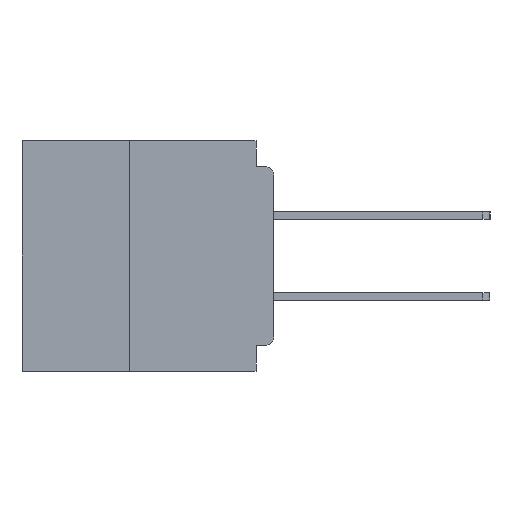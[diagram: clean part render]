
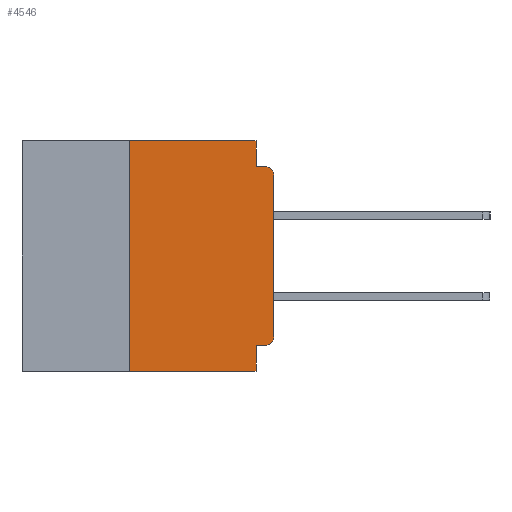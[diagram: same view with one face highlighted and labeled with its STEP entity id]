
A CAD part, left-side view. The second image highlights one B-rep face of the part: STEP entity #4546.
In plain terms, the highlighted planar face has unit normal (-1, 0, 0).
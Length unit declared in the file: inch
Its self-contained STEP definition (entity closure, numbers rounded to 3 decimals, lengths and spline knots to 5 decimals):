
#869 = EDGE_CURVE ( 'NONE', #6535, #37464, #2580, .T. ) ;
#2446 = CARTESIAN_POINT ( 'NONE',  ( 0., 0.015, -0.34 ) ) ;
#2580 = LINE ( 'NONE', #14426, #40283 ) ;
#2788 = CARTESIAN_POINT ( 'NONE',  ( 0., 0.031, -0.4 ) ) ;
#2924 = CARTESIAN_POINT ( 'NONE',  ( 0., 0., -0.045 ) ) ;
#3653 = EDGE_CURVE ( 'NONE', #5623, #40461, #44685, .T. ) ;
#4222 = DIRECTION ( 'NONE',  ( 0., 0., -1. ) ) ;
#4546 = ADVANCED_FACE ( 'NONE', ( #43431 ), #31111, .F. ) ;
#4682 = ORIENTED_EDGE ( 'NONE', *, *, #29597, .F. ) ;
#5073 = DIRECTION ( 'NONE',  ( 0., 0., 1. ) ) ;
#5623 = VERTEX_POINT ( 'NONE', #37972 ) ;
#5752 = LINE ( 'NONE', #2788, #24619 ) ;
#5848 = EDGE_CURVE ( 'NONE', #23133, #26638, #44466, .T. ) ;
#6273 = DIRECTION ( 'NONE',  ( 0., 0., -1. ) ) ;
#6535 = VERTEX_POINT ( 'NONE', #35737 ) ;
#7078 = ORIENTED_EDGE ( 'NONE', *, *, #17910, .T. ) ;
#7271 = CARTESIAN_POINT ( 'NONE',  ( 0., 0.015, -0.06 ) ) ;
#8165 = CARTESIAN_POINT ( 'NONE',  ( 0., 0.015, -0.355 ) ) ;
#8594 = DIRECTION ( 'NONE',  ( 1., 0., 0. ) ) ;
#9610 = DIRECTION ( 'NONE',  ( 0., 1., 0. ) ) ;
#9863 = ORIENTED_EDGE ( 'NONE', *, *, #44425, .F. ) ;
#10443 = LINE ( 'NONE', #32131, #40440 ) ;
#11064 = DIRECTION ( 'NONE',  ( 0., 0., -1. ) ) ;
#12725 = CARTESIAN_POINT ( 'NONE',  ( 0., 0.031, -0.045 ) ) ;
#12985 = VECTOR ( 'NONE', #4222, 39.37008 ) ;
#14413 = CARTESIAN_POINT ( 'NONE',  ( 0., 0.031, 0. ) ) ;
#14426 = CARTESIAN_POINT ( 'NONE',  ( 0., 0.437, -0.4 ) ) ;
#14863 = CIRCLE ( 'NONE', #47612, 0.015 ) ;
#15536 = EDGE_CURVE ( 'NONE', #40461, #44170, #42951, .T. ) ;
#15879 = VERTEX_POINT ( 'NONE', #25126 ) ;
#16099 = LINE ( 'NONE', #2924, #27312 ) ;
#17910 = EDGE_CURVE ( 'NONE', #26638, #42758, #18728, .T. ) ;
#18728 = CIRCLE ( 'NONE', #38274, 0.015 ) ;
#20523 = CARTESIAN_POINT ( 'NONE',  ( 0., 0., 0. ) ) ;
#21500 = CARTESIAN_POINT ( 'NONE',  ( 0., 0.437, 0. ) ) ;
#21781 = DIRECTION ( 'NONE',  ( 0., 0., -1. ) ) ;
#22965 = VECTOR ( 'NONE', #5073, 39.37008 ) ;
#23133 = VERTEX_POINT ( 'NONE', #34748 ) ;
#23736 = EDGE_LOOP ( 'NONE', ( #25271, #7078, #24298, #45502, #30914, #46798, #47444, #9863, #4682, #31792 ) ) ;
#24298 = ORIENTED_EDGE ( 'NONE', *, *, #31698, .F. ) ;
#24448 = VERTEX_POINT ( 'NONE', #8165 ) ;
#24619 = VECTOR ( 'NONE', #21781, 39.37008 ) ;
#24737 = CARTESIAN_POINT ( 'NONE',  ( 0., 0., -0.06 ) ) ;
#24789 = CARTESIAN_POINT ( 'NONE',  ( 0., 0.015, -0.045 ) ) ;
#25126 = CARTESIAN_POINT ( 'NONE',  ( 0., 0.031, -0.355 ) ) ;
#25271 = ORIENTED_EDGE ( 'NONE', *, *, #5848, .T. ) ;
#25281 = DIRECTION ( 'NONE',  ( 0., -1., 0. ) ) ;
#25521 = DIRECTION ( 'NONE',  ( 0., -1., 0. ) ) ;
#25658 = CARTESIAN_POINT ( 'NONE',  ( 0., 0.031, -0.4 ) ) ;
#25721 = VECTOR ( 'NONE', #46725, 39.37008 ) ;
#26638 = VERTEX_POINT ( 'NONE', #24737 ) ;
#27312 = VECTOR ( 'NONE', #25521, 39.37008 ) ;
#28806 = DIRECTION ( 'NONE',  ( -1., 0., 0. ) ) ;
#28875 = EDGE_CURVE ( 'NONE', #6535, #5623, #41717, .T. ) ;
#29597 = EDGE_CURVE ( 'NONE', #24448, #15879, #10443, .T. ) ;
#30914 = ORIENTED_EDGE ( 'NONE', *, *, #3653, .F. ) ;
#31111 = PLANE ( 'NONE',  #34516 ) ;
#31234 = DIRECTION ( 'NONE',  ( 0., -1., 0. ) ) ;
#31698 = EDGE_CURVE ( 'NONE', #44170, #42758, #16099, .T. ) ;
#31792 = ORIENTED_EDGE ( 'NONE', *, *, #46714, .T. ) ;
#32131 = CARTESIAN_POINT ( 'NONE',  ( 0., 0., -0.355 ) ) ;
#33562 = DIRECTION ( 'NONE',  ( -1., 0., 0. ) ) ;
#34170 = CARTESIAN_POINT ( 'NONE',  ( 0., 0.031, 0. ) ) ;
#34516 = AXIS2_PLACEMENT_3D ( 'NONE', #45983, #8594, #34895 ) ;
#34748 = CARTESIAN_POINT ( 'NONE',  ( 0., 0., -0.34 ) ) ;
#34895 = DIRECTION ( 'NONE',  ( 0., 0., -1. ) ) ;
#35166 = CARTESIAN_POINT ( 'NONE',  ( 0., 0.25, -0.4 ) ) ;
#35737 = CARTESIAN_POINT ( 'NONE',  ( 0., 0.25, -0.4 ) ) ;
#37464 = VERTEX_POINT ( 'NONE', #25658 ) ;
#37972 = CARTESIAN_POINT ( 'NONE',  ( 0., 0.25, 0. ) ) ;
#38274 = AXIS2_PLACEMENT_3D ( 'NONE', #7271, #33562, #11064 ) ;
#40283 = VECTOR ( 'NONE', #31234, 39.37008 ) ;
#40440 = VECTOR ( 'NONE', #9610, 39.37008 ) ;
#40461 = VERTEX_POINT ( 'NONE', #14413 ) ;
#41717 = LINE ( 'NONE', #35166, #22965 ) ;
#42758 = VERTEX_POINT ( 'NONE', #24789 ) ;
#42951 = LINE ( 'NONE', #34170, #12985 ) ;
#43431 = FACE_OUTER_BOUND ( 'NONE', #23736, .T. ) ;
#43532 = VECTOR ( 'NONE', #25281, 39.37008 ) ;
#44170 = VERTEX_POINT ( 'NONE', #12725 ) ;
#44425 = EDGE_CURVE ( 'NONE', #15879, #37464, #5752, .T. ) ;
#44466 = LINE ( 'NONE', #20523, #25721 ) ;
#44685 = LINE ( 'NONE', #21500, #43532 ) ;
#45502 = ORIENTED_EDGE ( 'NONE', *, *, #15536, .F. ) ;
#45983 = CARTESIAN_POINT ( 'NONE',  ( 0., 0.437, 0. ) ) ;
#46714 = EDGE_CURVE ( 'NONE', #24448, #23133, #14863, .T. ) ;
#46725 = DIRECTION ( 'NONE',  ( 0., 0., 1. ) ) ;
#46798 = ORIENTED_EDGE ( 'NONE', *, *, #28875, .F. ) ;
#47444 = ORIENTED_EDGE ( 'NONE', *, *, #869, .T. ) ;
#47612 = AXIS2_PLACEMENT_3D ( 'NONE', #2446, #28806, #6273 ) ;
